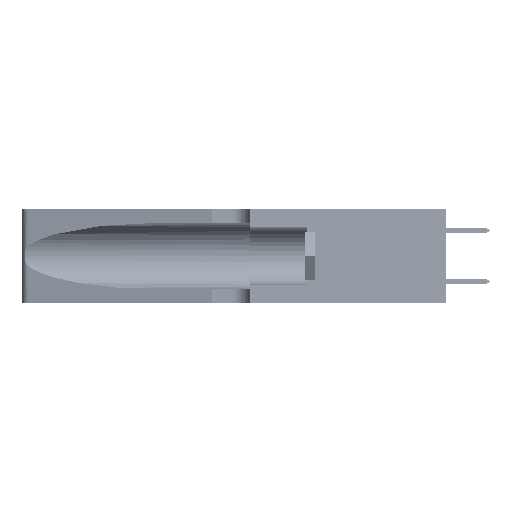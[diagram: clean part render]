
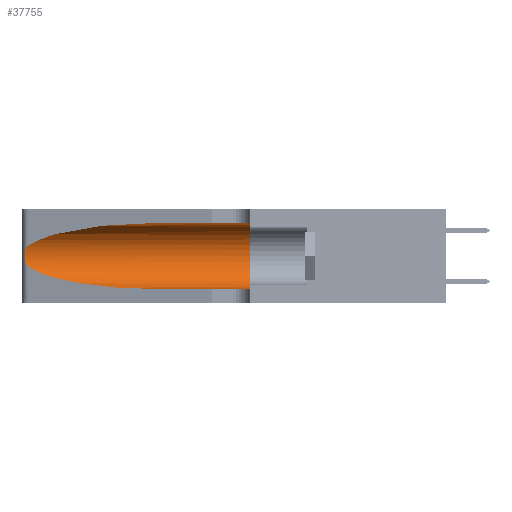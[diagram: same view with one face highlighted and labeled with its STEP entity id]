
A CAD part, left-side view. The second image highlights one B-rep face of the part: STEP entity #37755.
In plain terms, the highlighted cylindrical face has radius 3.308 mm (diameter 6.617 mm), a partial arc.
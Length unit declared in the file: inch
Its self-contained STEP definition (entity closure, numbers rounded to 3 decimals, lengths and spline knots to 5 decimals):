
#1 = CARTESIAN_POINT ( 'NONE',  ( 0.25487, 1.22718, 0.22369 ) ) ;
#237 = B_SPLINE_CURVE_WITH_KNOTS ( 'NONE', 3,
 ( #10792, #6861, #30066, #37945, #14719, #41893, #18572, #45773, #22464, #49653, #26350, #3087, #30233, #7033 ),
 .UNSPECIFIED., .F., .F.,
 ( 4, 2, 2, 2, 2, 2, 4 ),
 ( 0., 0.00027, 0.00053, 0.00107, 0.0016, 0.00187, 0.00214 ),
 .UNSPECIFIED. ) ;
#838 = EDGE_LOOP ( 'NONE', ( #37149, #47516, #1896, #26234, #28179, #8765 ) ) ;
#1377 = VERTEX_POINT ( 'NONE', #18759 ) ;
#1896 = ORIENTED_EDGE ( 'NONE', *, *, #46942, .T. ) ;
#3087 = CARTESIAN_POINT ( 'NONE',  ( 0.25639, 1.23186, 0.15144 ) ) ;
#5340 = CYLINDRICAL_SURFACE ( 'NONE', #15267, 0.13025 ) ;
#6006 = EDGE_CURVE ( 'NONE', #35894, #1377, #8711, .T. ) ;
#6550 = FACE_OUTER_BOUND ( 'NONE', #838, .T. ) ;
#6861 = CARTESIAN_POINT ( 'NONE',  ( 0.25555, 1.22994, 0.2215 ) ) ;
#7033 = CARTESIAN_POINT ( 'NONE',  ( 0.25487, 1.22718, 0.14631 ) ) ;
#7676 = CARTESIAN_POINT ( 'NONE',  ( 0.1305, 0.72297, 0.31525 ) ) ;
#8711 = LINE ( 'NONE', #48354, #48811 ) ;
#8765 = ORIENTED_EDGE ( 'NONE', *, *, #38246, .F. ) ;
#10792 = CARTESIAN_POINT ( 'NONE',  ( 0.25487, 1.22718, 0.22369 ) ) ;
#11425 = CARTESIAN_POINT ( 'NONE',  ( 0.1305, 1.61858, 0.31525 ) ) ;
#11932 = CARTESIAN_POINT ( 'NONE',  ( 0.1305, 0.72297, 0.05475 ) ) ;
#13880 = EDGE_CURVE ( 'NONE', #24082, #38778, #237, .T. ) ;
#14719 = CARTESIAN_POINT ( 'NONE',  ( 0.25854, 1.2359, 0.20912 ) ) ;
#15267 = AXIS2_PLACEMENT_3D ( 'NONE', #20420, #28205, #16563 ) ;
#15597 = CARTESIAN_POINT ( 'NONE',  ( 0.18966, 0.96281, 0.05475 ) ) ;
#16563 = DIRECTION ( 'NONE',  ( 0., 0., -1. ) ) ;
#16940 = AXIS2_PLACEMENT_3D ( 'NONE', #40440, #17137, #44332 ) ;
#17045 = EDGE_CURVE ( 'NONE', #20155, #24082, #33399, .T. ) ;
#17137 = DIRECTION ( 'NONE',  ( 0., 1., 0. ) ) ;
#17976 = EDGE_CURVE ( 'NONE', #36089, #1377, #23131, .T. ) ;
#18320 = CARTESIAN_POINT ( 'NONE',  ( 0.1305, 0.72297, 0.31525 ) ) ;
#18572 = CARTESIAN_POINT ( 'NONE',  ( 0.26075, 1.23896, 0.19203 ) ) ;
#18759 = CARTESIAN_POINT ( 'NONE',  ( 0.1305, 0.35, 0.05475 ) ) ;
#20155 = VERTEX_POINT ( 'NONE', #18320 ) ;
#20420 = CARTESIAN_POINT ( 'NONE',  ( 0.1305, 1.61858, 0.185 ) ) ;
#22464 = CARTESIAN_POINT ( 'NONE',  ( 0.26017, 1.23833, 0.17102 ) ) ;
#23110 = CARTESIAN_POINT ( 'NONE',  ( 0.18966, 0.96281, 0.31525 ) ) ;
#23131 = CIRCLE ( 'NONE', #16940, 0.13025 ) ;
#23274 = CARTESIAN_POINT ( 'NONE',  ( 0.2373, 1.15595, 0.28018 ) ) ;
#24052 = CARTESIAN_POINT ( 'NONE',  ( 0.25487, 1.22718, 0.22369 ) ) ;
#24082 = VERTEX_POINT ( 'NONE', #24052 ) ;
#25915 = CARTESIAN_POINT ( 'NONE',  ( 0.25487, 1.22718, 0.14631 ) ) ;
#26234 = ORIENTED_EDGE ( 'NONE', *, *, #6006, .T. ) ;
#26350 = CARTESIAN_POINT ( 'NONE',  ( 0.25789, 1.23486, 0.15765 ) ) ;
#27065 = DIRECTION ( 'NONE',  ( 0., -1., 0. ) ) ;
#27075 = CARTESIAN_POINT ( 'NONE',  ( 0.25487, 1.22718, 0.14631 ) ) ;
#28179 = ORIENTED_EDGE ( 'NONE', *, *, #17976, .F. ) ;
#28205 = DIRECTION ( 'NONE',  ( 0., -1., 0. ) ) ;
#30066 = CARTESIAN_POINT ( 'NONE',  ( 0.25639, 1.23184, 0.21858 ) ) ;
#30233 = CARTESIAN_POINT ( 'NONE',  ( 0.25555, 1.22993, 0.14849 ) ) ;
#32348 = CARTESIAN_POINT ( 'NONE',  ( 0.1305, 0.35, 0.31525 ) ) ;
#33399 =( BOUNDED_CURVE ( )  B_SPLINE_CURVE ( 3, ( #7676, #23110, #23274, #1 ),
 .UNSPECIFIED., .F., .F. ) 
 B_SPLINE_CURVE_WITH_KNOTS ( ( 4, 4 ),
 ( 1.5708, 2.84003 ),
 .UNSPECIFIED. ) 
 CURVE ( )  GEOMETRIC_REPRESENTATION_ITEM ( )  RATIONAL_B_SPLINE_CURVE ( ( 1., 0.87, 0.87, 1. ) ) 
 REPRESENTATION_ITEM ( '' )  );
#34582 = DIRECTION ( 'NONE',  ( 0., -1., 0. ) ) ;
#34692 =( BOUNDED_CURVE ( )  B_SPLINE_CURVE ( 3, ( #27075, #34849, #15597, #42764 ),
 .UNSPECIFIED., .F., .T. ) 
 B_SPLINE_CURVE_WITH_KNOTS ( ( 4, 4 ),
 ( 3.44316, 4.71239 ),
 .UNSPECIFIED. ) 
 CURVE ( )  GEOMETRIC_REPRESENTATION_ITEM ( )  RATIONAL_B_SPLINE_CURVE ( ( 1., 0.87, 0.87, 1. ) ) 
 REPRESENTATION_ITEM ( '' )  );
#34849 = CARTESIAN_POINT ( 'NONE',  ( 0.2373, 1.15595, 0.08982 ) ) ;
#35894 = VERTEX_POINT ( 'NONE', #11932 ) ;
#36089 = VERTEX_POINT ( 'NONE', #32348 ) ;
#36239 = LINE ( 'NONE', #11425, #45425 ) ;
#37149 = ORIENTED_EDGE ( 'NONE', *, *, #17045, .T. ) ;
#37755 = ADVANCED_FACE ( 'NONE', ( #6550 ), #5340, .F. ) ;
#37945 = CARTESIAN_POINT ( 'NONE',  ( 0.25787, 1.23484, 0.2124 ) ) ;
#38246 = EDGE_CURVE ( 'NONE', #20155, #36089, #36239, .T. ) ;
#38778 = VERTEX_POINT ( 'NONE', #25915 ) ;
#40440 = CARTESIAN_POINT ( 'NONE',  ( 0.1305, 0.35, 0.185 ) ) ;
#41893 = CARTESIAN_POINT ( 'NONE',  ( 0.26018, 1.23835, 0.19895 ) ) ;
#42764 = CARTESIAN_POINT ( 'NONE',  ( 0.1305, 0.72297, 0.05475 ) ) ;
#44332 = DIRECTION ( 'NONE',  ( 0., 0., 1. ) ) ;
#45425 = VECTOR ( 'NONE', #34582, 39.37008 ) ;
#45773 = CARTESIAN_POINT ( 'NONE',  ( 0.26075, 1.23896, 0.178 ) ) ;
#46942 = EDGE_CURVE ( 'NONE', #38778, #35894, #34692, .T. ) ;
#47516 = ORIENTED_EDGE ( 'NONE', *, *, #13880, .T. ) ;
#48354 = CARTESIAN_POINT ( 'NONE',  ( 0.1305, 1.61858, 0.05475 ) ) ;
#48811 = VECTOR ( 'NONE', #27065, 39.37008 ) ;
#49653 = CARTESIAN_POINT ( 'NONE',  ( 0.25856, 1.23593, 0.16098 ) ) ;
